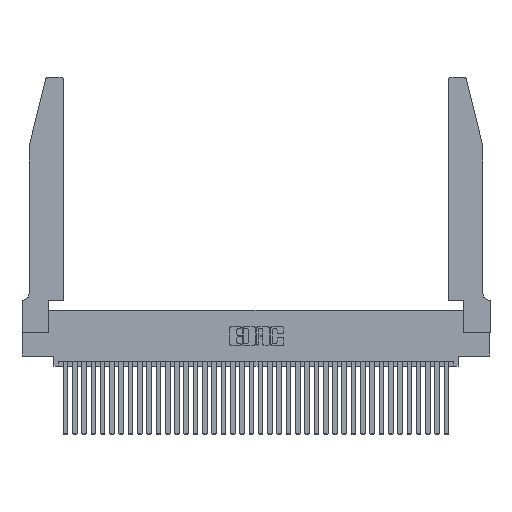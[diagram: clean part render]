
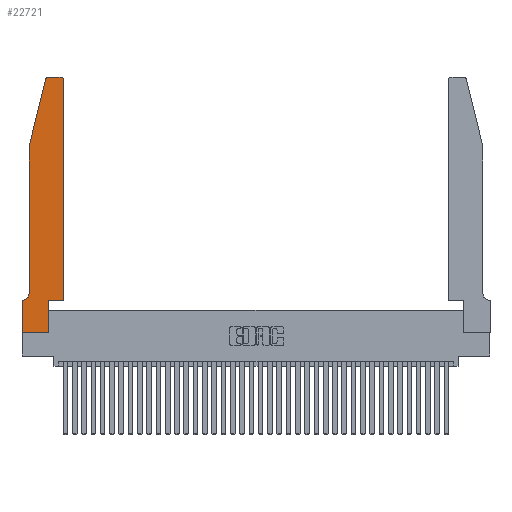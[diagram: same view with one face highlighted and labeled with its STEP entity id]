
A CAD part, top view. The second image highlights one B-rep face of the part: STEP entity #22721.
In plain terms, the highlighted planar face has unit normal (0, 0, 1).
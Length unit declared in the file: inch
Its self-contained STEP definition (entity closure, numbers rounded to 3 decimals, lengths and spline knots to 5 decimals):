
#37 = LINE ( 'NONE', #32169, #14659 ) ;
#427 = CARTESIAN_POINT ( 'NONE',  ( 0.0055, 0.35, 0.37 ) ) ;
#431 = DIRECTION ( 'NONE',  ( 0., -1., 0. ) ) ;
#556 = CARTESIAN_POINT ( 'NONE',  ( 0., 0., 0.37 ) ) ;
#729 = AXIS2_PLACEMENT_3D ( 'NONE', #23037, #5651, #26007 ) ;
#741 = VERTEX_POINT ( 'NONE', #18575 ) ;
#764 = DIRECTION ( 'NONE',  ( 0., 0., 1. ) ) ;
#809 = DIRECTION ( 'NONE',  ( 0., 0., 1. ) ) ;
#939 = CARTESIAN_POINT ( 'NONE',  ( 0.2865, 0.35, 0.37 ) ) ;
#1038 = CIRCLE ( 'NONE', #15538, 0.03 ) ;
#1462 = DIRECTION ( 'NONE',  ( -1., 0., 0. ) ) ;
#2372 = ORIENTED_EDGE ( 'NONE', *, *, #32924, .T. ) ;
#2639 = VERTEX_POINT ( 'NONE', #16343 ) ;
#3161 = CIRCLE ( 'NONE', #729, 0.07 ) ;
#3212 = DIRECTION ( 'NONE',  ( 1., 0., 0. ) ) ;
#3304 = ORIENTED_EDGE ( 'NONE', *, *, #27633, .T. ) ;
#3404 = CARTESIAN_POINT ( 'NONE',  ( 0.2605, 2.75, 0.37 ) ) ;
#3616 = ORIENTED_EDGE ( 'NONE', *, *, #9982, .T. ) ;
#4279 = EDGE_CURVE ( 'NONE', #20083, #18710, #31719, .T. ) ;
#4685 = CARTESIAN_POINT ( 'NONE',  ( 0.0755, 2., 0.37 ) ) ;
#4831 = EDGE_LOOP ( 'NONE', ( #2372, #19501, #7247, #29058, #17229, #6576, #27002, #3616, #16827, #19995, #35737, #3304 ) ) ;
#5651 = DIRECTION ( 'NONE',  ( 0., 0., -1. ) ) ;
#5959 = FACE_OUTER_BOUND ( 'NONE', #4831, .T. ) ;
#6330 = CARTESIAN_POINT ( 'NONE',  ( 0., 0., 0.37 ) ) ;
#6576 = ORIENTED_EDGE ( 'NONE', *, *, #20765, .T. ) ;
#6712 = DIRECTION ( 'NONE',  ( 0., 1., 0. ) ) ;
#7107 = EDGE_CURVE ( 'NONE', #25015, #741, #1038, .T. ) ;
#7199 = VECTOR ( 'NONE', #10581, 39.37008 ) ;
#7247 = ORIENTED_EDGE ( 'NONE', *, *, #36316, .T. ) ;
#7855 = EDGE_CURVE ( 'NONE', #32479, #2639, #13902, .T. ) ;
#8265 = LINE ( 'NONE', #25255, #30559 ) ;
#8525 = VECTOR ( 'NONE', #18368, 39.37008 ) ;
#8675 = LINE ( 'NONE', #16852, #30079 ) ;
#8903 = AXIS2_PLACEMENT_3D ( 'NONE', #31396, #13996, #34283 ) ;
#9482 = VERTEX_POINT ( 'NONE', #27553 ) ;
#9756 = VECTOR ( 'NONE', #1462, 39.37008 ) ;
#9982 = EDGE_CURVE ( 'NONE', #36625, #20083, #8265, .T. ) ;
#10581 = DIRECTION ( 'NONE',  ( -0.239, -0.971, 0. ) ) ;
#11681 = VERTEX_POINT ( 'NONE', #13306 ) ;
#12582 = VERTEX_POINT ( 'NONE', #26200 ) ;
#12583 = CARTESIAN_POINT ( 'NONE',  ( 0.4505, 0.35, 0.37 ) ) ;
#12984 = VECTOR ( 'NONE', #6712, 39.37008 ) ;
#13131 = CARTESIAN_POINT ( 'NONE',  ( 0.0755, 0.35, 0.37 ) ) ;
#13173 = CARTESIAN_POINT ( 'NONE',  ( 0.2865, 0., 0.37 ) ) ;
#13306 = CARTESIAN_POINT ( 'NONE',  ( 0., 0.35, 0.37 ) ) ;
#13902 = LINE ( 'NONE', #12583, #12984 ) ;
#13996 = DIRECTION ( 'NONE',  ( 0., 0., 1. ) ) ;
#14659 = VECTOR ( 'NONE', #35074, 39.37008 ) ;
#15538 = AXIS2_PLACEMENT_3D ( 'NONE', #18236, #809, #21158 ) ;
#16051 = VECTOR ( 'NONE', #23765, 39.37008 ) ;
#16343 = CARTESIAN_POINT ( 'NONE',  ( 0.4505, 2.72, 0.37 ) ) ;
#16588 = AXIS2_PLACEMENT_3D ( 'NONE', #35603, #764, #21113 ) ;
#16827 = ORIENTED_EDGE ( 'NONE', *, *, #4279, .T. ) ;
#16852 = CARTESIAN_POINT ( 'NONE',  ( 0.0755, 2., 0.37 ) ) ;
#16875 = EDGE_CURVE ( 'NONE', #35786, #12582, #8675, .T. ) ;
#17229 = ORIENTED_EDGE ( 'NONE', *, *, #35368, .T. ) ;
#17452 = LINE ( 'NONE', #13131, #9756 ) ;
#18189 = PLANE ( 'NONE',  #16588 ) ;
#18236 = CARTESIAN_POINT ( 'NONE',  ( 0.284, 2.72, 0.37 ) ) ;
#18368 = DIRECTION ( 'NONE',  ( 0., 1., 0. ) ) ;
#18575 = CARTESIAN_POINT ( 'NONE',  ( 0.25487, 2.72718, 0.37 ) ) ;
#18710 = VERTEX_POINT ( 'NONE', #22417 ) ;
#19501 = ORIENTED_EDGE ( 'NONE', *, *, #7107, .T. ) ;
#19995 = ORIENTED_EDGE ( 'NONE', *, *, #22184, .T. ) ;
#20083 = VERTEX_POINT ( 'NONE', #13173 ) ;
#20765 = EDGE_CURVE ( 'NONE', #24081, #11681, #17452, .T. ) ;
#21113 = DIRECTION ( 'NONE',  ( 1., 0., 0. ) ) ;
#21158 = DIRECTION ( 'NONE',  ( 1., 0., 0. ) ) ;
#22184 = EDGE_CURVE ( 'NONE', #18710, #32479, #37, .T. ) ;
#22417 = CARTESIAN_POINT ( 'NONE',  ( 0.2865, 0.35, 0.37 ) ) ;
#22721 = ADVANCED_FACE ( 'NONE', ( #5959 ), #18189, .T. ) ;
#22738 = LINE ( 'NONE', #556, #37275 ) ;
#23037 = CARTESIAN_POINT ( 'NONE',  ( 0.0055, 0.42, 0.37 ) ) ;
#23765 = DIRECTION ( 'NONE',  ( -1., 0., 0. ) ) ;
#24081 = VERTEX_POINT ( 'NONE', #427 ) ;
#25015 = VERTEX_POINT ( 'NONE', #28659 ) ;
#25255 = CARTESIAN_POINT ( 'NONE',  ( 0., 0., 0.37 ) ) ;
#26007 = DIRECTION ( 'NONE',  ( -1., 0., 0. ) ) ;
#26200 = CARTESIAN_POINT ( 'NONE',  ( 0.0755, 0.42, 0.37 ) ) ;
#27002 = ORIENTED_EDGE ( 'NONE', *, *, #27920, .T. ) ;
#27553 = CARTESIAN_POINT ( 'NONE',  ( 0.4205, 2.75, 0.37 ) ) ;
#27633 = EDGE_CURVE ( 'NONE', #2639, #9482, #32748, .T. ) ;
#27920 = EDGE_CURVE ( 'NONE', #11681, #36625, #22738, .T. ) ;
#28659 = CARTESIAN_POINT ( 'NONE',  ( 0.284, 2.75, 0.37 ) ) ;
#29058 = ORIENTED_EDGE ( 'NONE', *, *, #16875, .T. ) ;
#30079 = VECTOR ( 'NONE', #31475, 39.37008 ) ;
#30435 = LINE ( 'NONE', #4685, #7199 ) ;
#30559 = VECTOR ( 'NONE', #3212, 39.37008 ) ;
#30627 = LINE ( 'NONE', #3404, #16051 ) ;
#31396 = CARTESIAN_POINT ( 'NONE',  ( 0.4205, 2.72, 0.37 ) ) ;
#31475 = DIRECTION ( 'NONE',  ( 0., -1., 0. ) ) ;
#31719 = LINE ( 'NONE', #939, #8525 ) ;
#32169 = CARTESIAN_POINT ( 'NONE',  ( 0.4505, 0.35, 0.37 ) ) ;
#32479 = VERTEX_POINT ( 'NONE', #35588 ) ;
#32748 = CIRCLE ( 'NONE', #8903, 0.03 ) ;
#32924 = EDGE_CURVE ( 'NONE', #9482, #25015, #30627, .T. ) ;
#33803 = CARTESIAN_POINT ( 'NONE',  ( 0.0755, 2., 0.37 ) ) ;
#34283 = DIRECTION ( 'NONE',  ( 1., 0., 0. ) ) ;
#35074 = DIRECTION ( 'NONE',  ( 1., 0., 0. ) ) ;
#35368 = EDGE_CURVE ( 'NONE', #12582, #24081, #3161, .T. ) ;
#35588 = CARTESIAN_POINT ( 'NONE',  ( 0.4505, 0.35, 0.37 ) ) ;
#35603 = CARTESIAN_POINT ( 'NONE',  ( 0., 0.35, 0.37 ) ) ;
#35737 = ORIENTED_EDGE ( 'NONE', *, *, #7855, .T. ) ;
#35786 = VERTEX_POINT ( 'NONE', #33803 ) ;
#36316 = EDGE_CURVE ( 'NONE', #741, #35786, #30435, .T. ) ;
#36625 = VERTEX_POINT ( 'NONE', #6330 ) ;
#37275 = VECTOR ( 'NONE', #431, 39.37008 ) ;
